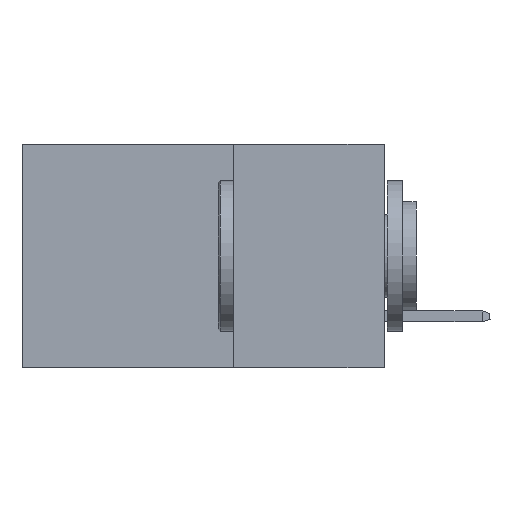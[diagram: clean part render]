
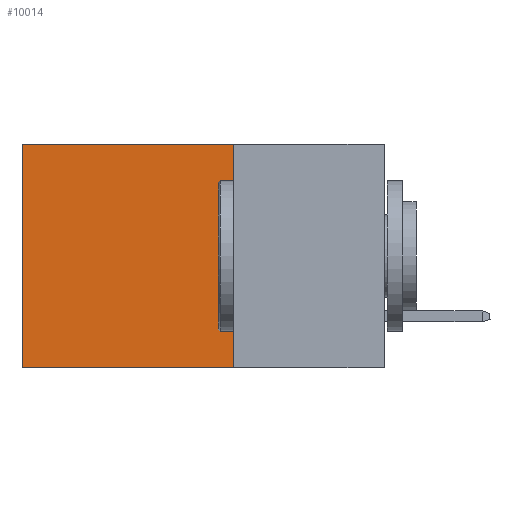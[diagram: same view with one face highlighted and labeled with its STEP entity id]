
A CAD part, left-side view. The second image highlights one B-rep face of the part: STEP entity #10014.
In plain terms, the highlighted planar face has unit normal (-1, 0, 0).
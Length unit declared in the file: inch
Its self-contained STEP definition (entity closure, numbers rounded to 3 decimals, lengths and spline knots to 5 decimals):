
#113 = VECTOR ( 'NONE', #9977, 39.37008 ) ;
#692 = DIRECTION ( 'NONE',  ( 1., 0., 0. ) ) ;
#798 = AXIS2_PLACEMENT_3D ( 'NONE', #2272, #692, #7073 ) ;
#1137 = VECTOR ( 'NONE', #2035, 39.37008 ) ;
#1219 = LINE ( 'NONE', #9833, #9080 ) ;
#1770 = ORIENTED_EDGE ( 'NONE', *, *, #4225, .F. ) ;
#2035 = DIRECTION ( 'NONE',  ( 0., 1., 0. ) ) ;
#2092 = VERTEX_POINT ( 'NONE', #8531 ) ;
#2098 = CARTESIAN_POINT ( 'NONE',  ( 0.298, 0.6, 0. ) ) ;
#2272 = CARTESIAN_POINT ( 'NONE',  ( 0.298, 0.25, 0. ) ) ;
#2545 = EDGE_CURVE ( 'NONE', #3995, #2956, #9754, .T. ) ;
#2818 = EDGE_LOOP ( 'NONE', ( #4809, #5889, #1770, #4427 ) ) ;
#2956 = VERTEX_POINT ( 'NONE', #4232 ) ;
#3136 = LINE ( 'NONE', #2098, #6691 ) ;
#3630 = FACE_OUTER_BOUND ( 'NONE', #2818, .T. ) ;
#3995 = VERTEX_POINT ( 'NONE', #7215 ) ;
#4225 = EDGE_CURVE ( 'NONE', #2092, #3995, #4373, .T. ) ;
#4232 = CARTESIAN_POINT ( 'NONE',  ( 0.298, 0.6, -0.37 ) ) ;
#4373 = LINE ( 'NONE', #8342, #113 ) ;
#4427 = ORIENTED_EDGE ( 'NONE', *, *, #10344, .T. ) ;
#4809 = ORIENTED_EDGE ( 'NONE', *, *, #9915, .T. ) ;
#5079 = CARTESIAN_POINT ( 'NONE',  ( 0.298, 0.6, 0. ) ) ;
#5889 = ORIENTED_EDGE ( 'NONE', *, *, #2545, .F. ) ;
#6089 = DIRECTION ( 'NONE',  ( 0., 0., -1. ) ) ;
#6691 = VECTOR ( 'NONE', #6089, 39.37008 ) ;
#7073 = DIRECTION ( 'NONE',  ( 0., 0., -1. ) ) ;
#7215 = CARTESIAN_POINT ( 'NONE',  ( 0.298, 0.25, -0.37 ) ) ;
#8342 = CARTESIAN_POINT ( 'NONE',  ( 0.298, 0.25, 0. ) ) ;
#8531 = CARTESIAN_POINT ( 'NONE',  ( 0.298, 0.25, 0. ) ) ;
#8830 = PLANE ( 'NONE',  #798 ) ;
#9080 = VECTOR ( 'NONE', #9969, 39.37008 ) ;
#9754 = LINE ( 'NONE', #10022, #1137 ) ;
#9833 = CARTESIAN_POINT ( 'NONE',  ( 0.298, 0.25, 0. ) ) ;
#9915 = EDGE_CURVE ( 'NONE', #10320, #2956, #3136, .T. ) ;
#9969 = DIRECTION ( 'NONE',  ( 0., 1., 0. ) ) ;
#9977 = DIRECTION ( 'NONE',  ( 0., 0., -1. ) ) ;
#10014 = ADVANCED_FACE ( 'NONE', ( #3630 ), #8830, .F. ) ;
#10022 = CARTESIAN_POINT ( 'NONE',  ( 0.298, 0.25, -0.37 ) ) ;
#10320 = VERTEX_POINT ( 'NONE', #5079 ) ;
#10344 = EDGE_CURVE ( 'NONE', #2092, #10320, #1219, .T. ) ;
